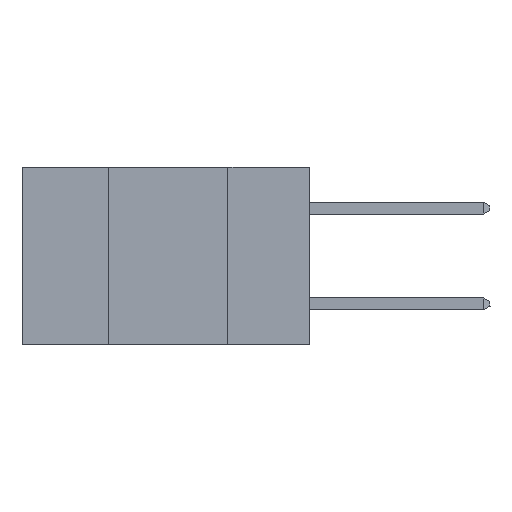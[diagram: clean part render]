
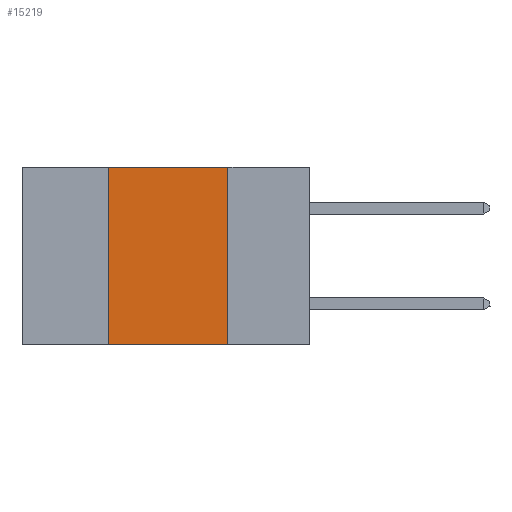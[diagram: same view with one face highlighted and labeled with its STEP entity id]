
A CAD part, left-side view. The second image highlights one B-rep face of the part: STEP entity #15219.
In plain terms, the highlighted planar face has unit normal (-1, 0, 0).
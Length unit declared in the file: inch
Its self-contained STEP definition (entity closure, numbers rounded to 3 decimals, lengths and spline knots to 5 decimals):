
#317 = ORIENTED_EDGE ( 'NONE', *, *, #13007, .F. ) ;
#2161 = EDGE_LOOP ( 'NONE', ( #9496, #21393, #317, #18257 ) ) ;
#2951 = CARTESIAN_POINT ( 'NONE',  ( 0., 0.17, 0. ) ) ;
#3105 = DIRECTION ( 'NONE',  ( 1., 0., 0. ) ) ;
#3759 = AXIS2_PLACEMENT_3D ( 'NONE', #13350, #3105, #7868 ) ;
#4072 = LINE ( 'NONE', #19501, #21709 ) ;
#4275 = LINE ( 'NONE', #17025, #21925 ) ;
#4724 = PLANE ( 'NONE',  #3759 ) ;
#7264 = CARTESIAN_POINT ( 'NONE',  ( 0., 0.42, 0. ) ) ;
#7868 = DIRECTION ( 'NONE',  ( 0., 0., -1. ) ) ;
#7881 = DIRECTION ( 'NONE',  ( 0., 0., -1. ) ) ;
#8215 = FACE_OUTER_BOUND ( 'NONE', #2161, .T. ) ;
#9496 = ORIENTED_EDGE ( 'NONE', *, *, #20579, .F. ) ;
#9913 = VERTEX_POINT ( 'NONE', #2951 ) ;
#11140 = EDGE_CURVE ( 'NONE', #15367, #9913, #4275, .T. ) ;
#11273 = CARTESIAN_POINT ( 'NONE',  ( 0., 0.6, -0.37 ) ) ;
#12018 = LINE ( 'NONE', #15364, #17587 ) ;
#12638 = EDGE_CURVE ( 'NONE', #19868, #22012, #21898, .T. ) ;
#13007 = EDGE_CURVE ( 'NONE', #19868, #15367, #12018, .T. ) ;
#13350 = CARTESIAN_POINT ( 'NONE',  ( 0., 0.6, 0. ) ) ;
#13442 = CARTESIAN_POINT ( 'NONE',  ( 0., 0.17, -0.37 ) ) ;
#13804 = DIRECTION ( 'NONE',  ( 0., 0., 1. ) ) ;
#15091 = DIRECTION ( 'NONE',  ( 0., -1., 0. ) ) ;
#15219 = ADVANCED_FACE ( 'NONE', ( #8215 ), #4724, .F. ) ;
#15223 = VECTOR ( 'NONE', #19730, 39.37008 ) ;
#15364 = CARTESIAN_POINT ( 'NONE',  ( 0., 0.42, 0. ) ) ;
#15367 = VERTEX_POINT ( 'NONE', #7264 ) ;
#17025 = CARTESIAN_POINT ( 'NONE',  ( 0., 0.6, 0. ) ) ;
#17587 = VECTOR ( 'NONE', #13804, 39.37008 ) ;
#18257 = ORIENTED_EDGE ( 'NONE', *, *, #12638, .T. ) ;
#19501 = CARTESIAN_POINT ( 'NONE',  ( 0., 0.17, 0. ) ) ;
#19730 = DIRECTION ( 'NONE',  ( 0., -1., 0. ) ) ;
#19868 = VERTEX_POINT ( 'NONE', #21094 ) ;
#20579 = EDGE_CURVE ( 'NONE', #9913, #22012, #4072, .T. ) ;
#21094 = CARTESIAN_POINT ( 'NONE',  ( 0., 0.42, -0.37 ) ) ;
#21393 = ORIENTED_EDGE ( 'NONE', *, *, #11140, .F. ) ;
#21709 = VECTOR ( 'NONE', #7881, 39.37008 ) ;
#21898 = LINE ( 'NONE', #11273, #15223 ) ;
#21925 = VECTOR ( 'NONE', #15091, 39.37008 ) ;
#22012 = VERTEX_POINT ( 'NONE', #13442 ) ;
